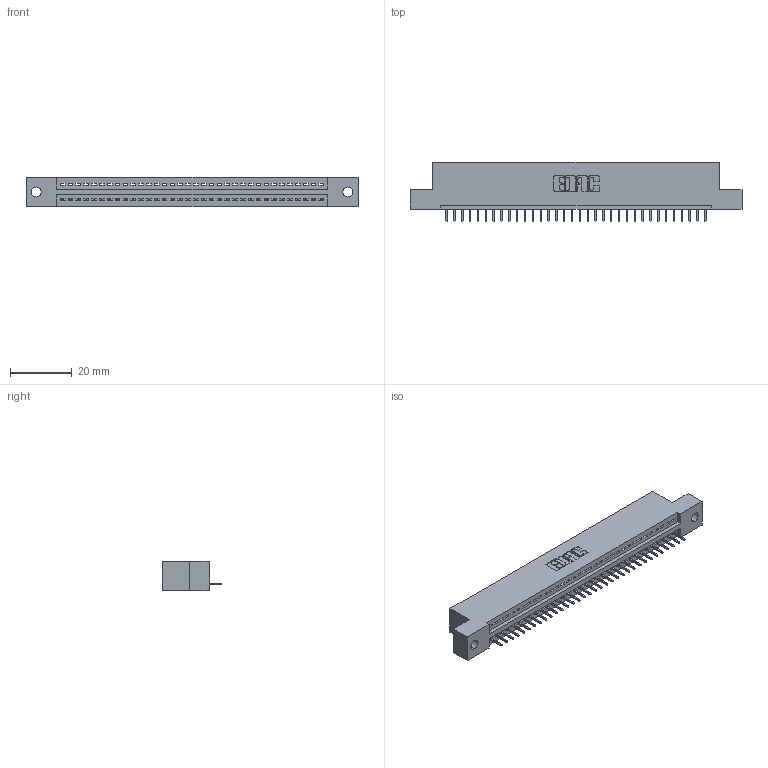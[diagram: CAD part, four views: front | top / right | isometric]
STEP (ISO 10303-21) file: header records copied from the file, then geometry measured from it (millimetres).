
FILE_DESCRIPTION (( 'STEP AP203' ), '1' );
FILE_NAME ('395-034-524-102.STEP', '2019-10-19T17:18:57', ( '' ), ( '' ), 'SwSTEP 2.0', 'SolidWorks 2016', '' );
FILE_SCHEMA (( 'CONFIG_CONTROL_DESIGN' ));
Length unit declared in the file: inch
Products named in the file (3): 345 Part_Flush Mounting Lugs - 0.128 Dia; 395-034-524-102; 345-292-001_345-293-124
Assembly tree (35 placements, depth 2):
  395-034-524-102
    345 Part_Flush Mounting Lugs - 0.128 Dia
    345-292-001_345-293-124  x34
Bounding box: 107.57 x 19.35 x 9.4 mm (x, y, z)
Volume: 9980.5 mm3; surface area: 12453.5 mm2
Topology: 35 solids, 35 shells, 2234 faces, 6461 edges, 4170 vertices
Faces by surface type: plane 1644, cylinder 590
Entity records: 26743 total; most frequent: CARTESIAN_POINT 4638, ORIENTED_EDGE 4606, DIRECTION 4063, EDGE_CURVE 2303, VECTOR 2039, LINE 2039, VERTEX_POINT 1530, AXIS2_PLACEMENT_3D 1012
